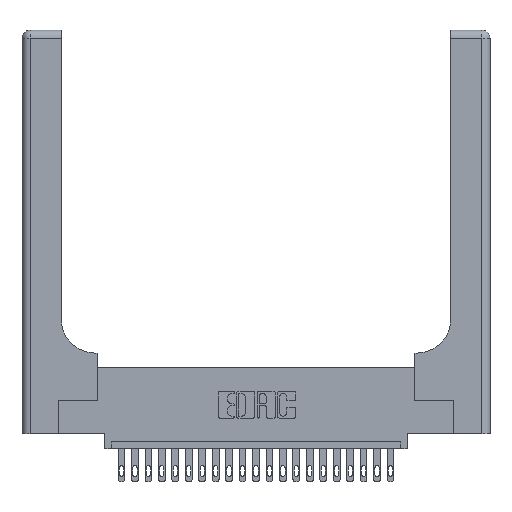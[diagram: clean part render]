
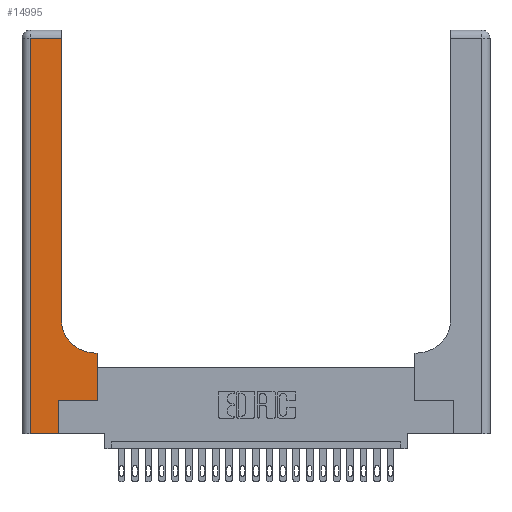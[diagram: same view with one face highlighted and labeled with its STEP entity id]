
A CAD part, top view. The second image highlights one B-rep face of the part: STEP entity #14995.
In plain terms, the highlighted planar face has unit normal (0, 0, 1).
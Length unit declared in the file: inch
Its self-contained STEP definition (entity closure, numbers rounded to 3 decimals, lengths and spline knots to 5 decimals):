
#97 = CARTESIAN_POINT ( 'NONE',  ( 0.2915, 2.94, 0.37 ) ) ;
#566 = VECTOR ( 'NONE', #7932, 39.37008 ) ;
#588 = VECTOR ( 'NONE', #10239, 39.37008 ) ;
#1027 = VERTEX_POINT ( 'NONE', #13816 ) ;
#1200 = VECTOR ( 'NONE', #19034, 39.37008 ) ;
#1297 = DIRECTION ( 'NONE',  ( 0., 1., 0. ) ) ;
#1515 = CARTESIAN_POINT ( 'NONE',  ( 0.5585, 0.25, 0.37 ) ) ;
#1770 = AXIS2_PLACEMENT_3D ( 'NONE', #2057, #14985, #5762 ) ;
#2057 = CARTESIAN_POINT ( 'NONE',  ( 0.5415, 0.85, 0.37 ) ) ;
#2067 = VERTEX_POINT ( 'NONE', #1515 ) ;
#2269 = ORIENTED_EDGE ( 'NONE', *, *, #7440, .T. ) ;
#3721 = VECTOR ( 'NONE', #18348, 39.37008 ) ;
#3943 = DIRECTION ( 'NONE',  ( -1., 0., 0. ) ) ;
#4286 = ORIENTED_EDGE ( 'NONE', *, *, #9593, .T. ) ;
#4414 = LINE ( 'NONE', #16152, #18946 ) ;
#4993 = LINE ( 'NONE', #13887, #9603 ) ;
#5097 = CARTESIAN_POINT ( 'NONE',  ( 0.06, 2.94, 0.37 ) ) ;
#5302 = CARTESIAN_POINT ( 'NONE',  ( 0.269, 0., 0.37 ) ) ;
#5438 = FACE_OUTER_BOUND ( 'NONE', #19091, .T. ) ;
#5556 = CARTESIAN_POINT ( 'NONE',  ( 0., 0., 0.37 ) ) ;
#5736 = ORIENTED_EDGE ( 'NONE', *, *, #10367, .T. ) ;
#5762 = DIRECTION ( 'NONE',  ( 1., 0., 0. ) ) ;
#5830 = DIRECTION ( 'NONE',  ( 0., -1., 0. ) ) ;
#6023 = ORIENTED_EDGE ( 'NONE', *, *, #7671, .T. ) ;
#6047 = VERTEX_POINT ( 'NONE', #20341 ) ;
#6314 = CARTESIAN_POINT ( 'NONE',  ( 0.269, 0.25, 0.37 ) ) ;
#7137 = CIRCLE ( 'NONE', #1770, 0.25 ) ;
#7440 = EDGE_CURVE ( 'NONE', #17005, #22810, #13004, .T. ) ;
#7530 = CARTESIAN_POINT ( 'NONE',  ( 0., 3., 0.37 ) ) ;
#7671 = EDGE_CURVE ( 'NONE', #16569, #2067, #21624, .T. ) ;
#7755 = ORIENTED_EDGE ( 'NONE', *, *, #15821, .T. ) ;
#7932 = DIRECTION ( 'NONE',  ( 1., 0., 0. ) ) ;
#8394 = DIRECTION ( 'NONE',  ( 0., 1., 0. ) ) ;
#8935 = DIRECTION ( 'NONE',  ( 0., 1., 0. ) ) ;
#9383 = DIRECTION ( 'NONE',  ( 0., 0., -1. ) ) ;
#9593 = EDGE_CURVE ( 'NONE', #1027, #11210, #4414, .T. ) ;
#9603 = VECTOR ( 'NONE', #8394, 39.37008 ) ;
#10239 = DIRECTION ( 'NONE',  ( -1., 0., 0. ) ) ;
#10367 = EDGE_CURVE ( 'NONE', #2067, #6047, #4993, .T. ) ;
#10410 = LINE ( 'NONE', #5556, #3721 ) ;
#11210 = VERTEX_POINT ( 'NONE', #97 ) ;
#11326 = ORIENTED_EDGE ( 'NONE', *, *, #21125, .T. ) ;
#12168 = VERTEX_POINT ( 'NONE', #20023 ) ;
#12688 = VERTEX_POINT ( 'NONE', #5302 ) ;
#12787 = CARTESIAN_POINT ( 'NONE',  ( 0.269, 0.25, 0.37 ) ) ;
#13004 = LINE ( 'NONE', #15059, #23070 ) ;
#13116 = ORIENTED_EDGE ( 'NONE', *, *, #20587, .T. ) ;
#13816 = CARTESIAN_POINT ( 'NONE',  ( 0.2915, 0.85, 0.37 ) ) ;
#13854 = VECTOR ( 'NONE', #8935, 39.37008 ) ;
#13887 = CARTESIAN_POINT ( 'NONE',  ( 0.5585, 0.25, 0.37 ) ) ;
#14136 = LINE ( 'NONE', #23320, #588 ) ;
#14296 = AXIS2_PLACEMENT_3D ( 'NONE', #7530, #9383, #3943 ) ;
#14985 = DIRECTION ( 'NONE',  ( 0., 0., -1. ) ) ;
#14995 = ADVANCED_FACE ( 'NONE', ( #5438 ), #15123, .F. ) ;
#15003 = ORIENTED_EDGE ( 'NONE', *, *, #20941, .T. ) ;
#15012 = LINE ( 'NONE', #20029, #13854 ) ;
#15059 = CARTESIAN_POINT ( 'NONE',  ( 0.06, 3., 0.37 ) ) ;
#15123 = PLANE ( 'NONE',  #14296 ) ;
#15821 = EDGE_CURVE ( 'NONE', #12168, #1027, #7137, .T. ) ;
#16152 = CARTESIAN_POINT ( 'NONE',  ( 0.2915, 3., 0.37 ) ) ;
#16569 = VERTEX_POINT ( 'NONE', #12787 ) ;
#17005 = VERTEX_POINT ( 'NONE', #5097 ) ;
#18348 = DIRECTION ( 'NONE',  ( 1., 0., 0. ) ) ;
#18946 = VECTOR ( 'NONE', #1297, 39.37008 ) ;
#19034 = DIRECTION ( 'NONE',  ( -1., 0., 0. ) ) ;
#19091 = EDGE_LOOP ( 'NONE', ( #4286, #15003, #2269, #13116, #11326, #6023, #5736, #20808, #7755 ) ) ;
#20023 = CARTESIAN_POINT ( 'NONE',  ( 0.5415, 0.6, 0.37 ) ) ;
#20029 = CARTESIAN_POINT ( 'NONE',  ( 0.269, 0., 0.37 ) ) ;
#20272 = LINE ( 'NONE', #21117, #1200 ) ;
#20320 = EDGE_CURVE ( 'NONE', #6047, #12168, #20272, .T. ) ;
#20341 = CARTESIAN_POINT ( 'NONE',  ( 0.5585, 0.6, 0.37 ) ) ;
#20587 = EDGE_CURVE ( 'NONE', #22810, #12688, #10410, .T. ) ;
#20808 = ORIENTED_EDGE ( 'NONE', *, *, #20320, .T. ) ;
#20941 = EDGE_CURVE ( 'NONE', #11210, #17005, #14136, .T. ) ;
#21117 = CARTESIAN_POINT ( 'NONE',  ( 0.2915, 0.6, 0.37 ) ) ;
#21125 = EDGE_CURVE ( 'NONE', #12688, #16569, #15012, .T. ) ;
#21624 = LINE ( 'NONE', #6314, #566 ) ;
#22810 = VERTEX_POINT ( 'NONE', #23480 ) ;
#23070 = VECTOR ( 'NONE', #5830, 39.37008 ) ;
#23320 = CARTESIAN_POINT ( 'NONE',  ( 0., 2.94, 0.37 ) ) ;
#23480 = CARTESIAN_POINT ( 'NONE',  ( 0.06, 0., 0.37 ) ) ;
